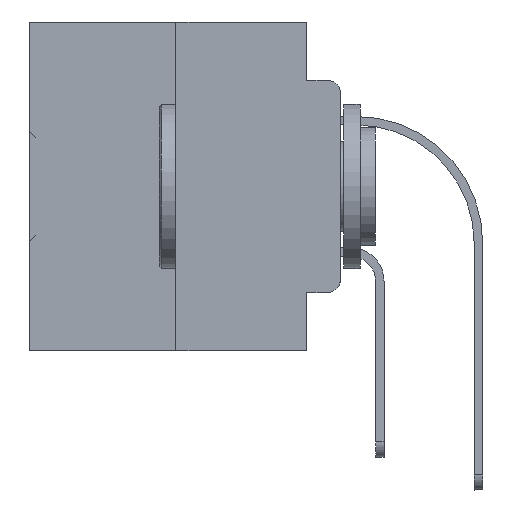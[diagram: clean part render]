
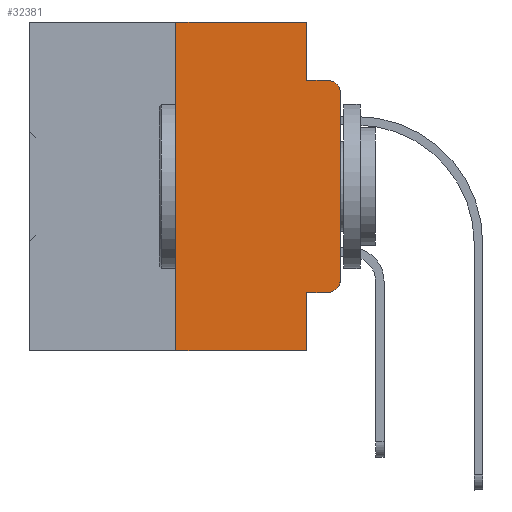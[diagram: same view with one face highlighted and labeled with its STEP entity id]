
A CAD part, left-side view. The second image highlights one B-rep face of the part: STEP entity #32381.
In plain terms, the highlighted planar face has unit normal (-1, 0, 0).
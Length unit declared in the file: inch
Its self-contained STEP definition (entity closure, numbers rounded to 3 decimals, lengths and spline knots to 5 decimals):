
#168 = LINE ( 'NONE', #25393, #14468 ) ;
#2033 = CARTESIAN_POINT ( 'NONE',  ( 0., 0.051, 0. ) ) ;
#2045 = ORIENTED_EDGE ( 'NONE', *, *, #20970, .F. ) ;
#2324 = VECTOR ( 'NONE', #39125, 39.37008 ) ;
#3124 = LINE ( 'NONE', #15420, #38953 ) ;
#3202 = EDGE_CURVE ( 'NONE', #34182, #8572, #28138, .T. ) ;
#3840 = LINE ( 'NONE', #25643, #27168 ) ;
#5666 = DIRECTION ( 'NONE',  ( 0., 0., -1. ) ) ;
#6700 = CARTESIAN_POINT ( 'NONE',  ( 0., 0.051, 0. ) ) ;
#6750 = AXIS2_PLACEMENT_3D ( 'NONE', #39450, #36419, #33386 ) ;
#6970 = VERTEX_POINT ( 'NONE', #34234 ) ;
#7242 = PLANE ( 'NONE',  #25373 ) ;
#8489 = CARTESIAN_POINT ( 'NONE',  ( 0., 0.02, -0.3915 ) ) ;
#8572 = VERTEX_POINT ( 'NONE', #26626 ) ;
#8591 = DIRECTION ( 'NONE',  ( 0., -1., 0. ) ) ;
#9255 = CARTESIAN_POINT ( 'NONE',  ( 0., 0.02, -0.0885 ) ) ;
#10632 = CARTESIAN_POINT ( 'NONE',  ( 0., 0.25, 0. ) ) ;
#10771 = VERTEX_POINT ( 'NONE', #23505 ) ;
#11154 = ORIENTED_EDGE ( 'NONE', *, *, #27075, .F. ) ;
#11506 = DIRECTION ( 'NONE',  ( -1., 0., 0. ) ) ;
#11569 = EDGE_CURVE ( 'NONE', #6970, #29354, #3124, .T. ) ;
#13267 = LINE ( 'NONE', #21961, #25495 ) ;
#13911 = EDGE_CURVE ( 'NONE', #36283, #34182, #22007, .T. ) ;
#14342 = EDGE_CURVE ( 'NONE', #36283, #29354, #168, .T. ) ;
#14468 = VECTOR ( 'NONE', #18301, 39.37008 ) ;
#15420 = CARTESIAN_POINT ( 'NONE',  ( 0., 0.473, -0.5 ) ) ;
#15575 = VERTEX_POINT ( 'NONE', #6700 ) ;
#16015 = CARTESIAN_POINT ( 'NONE',  ( 0., 0.473, 0. ) ) ;
#16335 = ORIENTED_EDGE ( 'NONE', *, *, #11569, .T. ) ;
#16351 = ORIENTED_EDGE ( 'NONE', *, *, #13911, .T. ) ;
#17923 = ORIENTED_EDGE ( 'NONE', *, *, #14342, .F. ) ;
#18301 = DIRECTION ( 'NONE',  ( 0., 0., -1. ) ) ;
#19136 = CARTESIAN_POINT ( 'NONE',  ( 0., 0.473, 0. ) ) ;
#19772 = VERTEX_POINT ( 'NONE', #22984 ) ;
#20730 = LINE ( 'NONE', #39710, #2324 ) ;
#20970 = EDGE_CURVE ( 'NONE', #19772, #24170, #3840, .T. ) ;
#21961 = CARTESIAN_POINT ( 'NONE',  ( 0., 0., 0. ) ) ;
#22007 = LINE ( 'NONE', #31485, #35112 ) ;
#22594 = DIRECTION ( 'NONE',  ( 0., -1., 0. ) ) ;
#22984 = CARTESIAN_POINT ( 'NONE',  ( 0., 0.051, -0.0885 ) ) ;
#23505 = CARTESIAN_POINT ( 'NONE',  ( 0., 0., -0.1085 ) ) ;
#23827 = DIRECTION ( 'NONE',  ( 0., 0., -1. ) ) ;
#24001 = CARTESIAN_POINT ( 'NONE',  ( 0., 0.02, -0.4115 ) ) ;
#24170 = VERTEX_POINT ( 'NONE', #9255 ) ;
#24407 = ORIENTED_EDGE ( 'NONE', *, *, #27713, .F. ) ;
#25037 = ORIENTED_EDGE ( 'NONE', *, *, #35035, .T. ) ;
#25373 = AXIS2_PLACEMENT_3D ( 'NONE', #19136, #28234, #31457 ) ;
#25393 = CARTESIAN_POINT ( 'NONE',  ( 0., 0.051, 0. ) ) ;
#25495 = VECTOR ( 'NONE', #37710, 39.37008 ) ;
#25643 = CARTESIAN_POINT ( 'NONE',  ( 0., 0.051, -0.0885 ) ) ;
#26626 = CARTESIAN_POINT ( 'NONE',  ( 0., 0., -0.3915 ) ) ;
#26888 = VECTOR ( 'NONE', #5666, 39.37008 ) ;
#27075 = EDGE_CURVE ( 'NONE', #6970, #33109, #20730, .T. ) ;
#27168 = VECTOR ( 'NONE', #22594, 39.37008 ) ;
#27522 = DIRECTION ( 'NONE',  ( 0., -1., 0. ) ) ;
#27713 = EDGE_CURVE ( 'NONE', #33109, #15575, #27917, .T. ) ;
#27917 = LINE ( 'NONE', #16015, #37170 ) ;
#28138 = CIRCLE ( 'NONE', #39115, 0.02 ) ;
#28234 = DIRECTION ( 'NONE',  ( 1., 0., 0. ) ) ;
#29247 = CARTESIAN_POINT ( 'NONE',  ( 0., 0.051, -0.5 ) ) ;
#29354 = VERTEX_POINT ( 'NONE', #29247 ) ;
#31081 = DIRECTION ( 'NONE',  ( 0., -1., 0. ) ) ;
#31249 = FACE_OUTER_BOUND ( 'NONE', #38035, .T. ) ;
#31457 = DIRECTION ( 'NONE',  ( 0., 0., -1. ) ) ;
#31485 = CARTESIAN_POINT ( 'NONE',  ( 0., 0.051, -0.4115 ) ) ;
#32381 = ADVANCED_FACE ( 'NONE', ( #31249 ), #7242, .F. ) ;
#33109 = VERTEX_POINT ( 'NONE', #10632 ) ;
#33312 = LINE ( 'NONE', #2033, #26888 ) ;
#33386 = DIRECTION ( 'NONE',  ( 0., 0., -1. ) ) ;
#33762 = ORIENTED_EDGE ( 'NONE', *, *, #3202, .T. ) ;
#33837 = CIRCLE ( 'NONE', #6750, 0.02 ) ;
#34182 = VERTEX_POINT ( 'NONE', #24001 ) ;
#34234 = CARTESIAN_POINT ( 'NONE',  ( 0., 0.25, -0.5 ) ) ;
#34877 = ORIENTED_EDGE ( 'NONE', *, *, #37495, .F. ) ;
#35035 = EDGE_CURVE ( 'NONE', #10771, #24170, #33837, .T. ) ;
#35112 = VECTOR ( 'NONE', #31081, 39.37008 ) ;
#35589 = EDGE_CURVE ( 'NONE', #8572, #10771, #13267, .T. ) ;
#35640 = CARTESIAN_POINT ( 'NONE',  ( 0., 0.051, -0.4115 ) ) ;
#35803 = ORIENTED_EDGE ( 'NONE', *, *, #35589, .T. ) ;
#36283 = VERTEX_POINT ( 'NONE', #35640 ) ;
#36419 = DIRECTION ( 'NONE',  ( -1., 0., 0. ) ) ;
#37170 = VECTOR ( 'NONE', #27522, 39.37008 ) ;
#37495 = EDGE_CURVE ( 'NONE', #15575, #19772, #33312, .T. ) ;
#37710 = DIRECTION ( 'NONE',  ( 0., 0., 1. ) ) ;
#38035 = EDGE_LOOP ( 'NONE', ( #35803, #25037, #2045, #34877, #24407, #11154, #16335, #17923, #16351, #33762 ) ) ;
#38953 = VECTOR ( 'NONE', #8591, 39.37008 ) ;
#39115 = AXIS2_PLACEMENT_3D ( 'NONE', #8489, #11506, #23827 ) ;
#39125 = DIRECTION ( 'NONE',  ( 0., 0., 1. ) ) ;
#39450 = CARTESIAN_POINT ( 'NONE',  ( 0., 0.02, -0.1085 ) ) ;
#39710 = CARTESIAN_POINT ( 'NONE',  ( 0., 0.25, 0. ) ) ;
